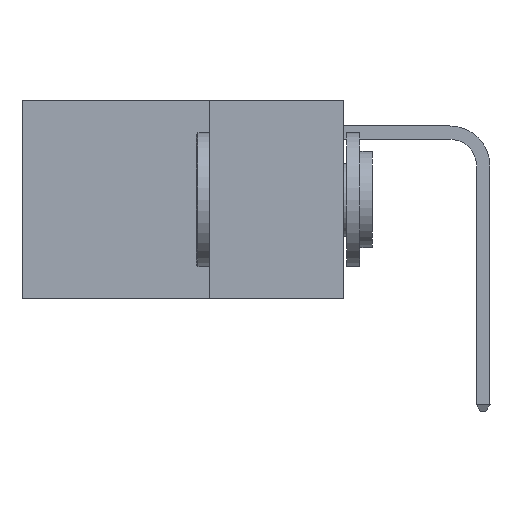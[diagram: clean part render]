
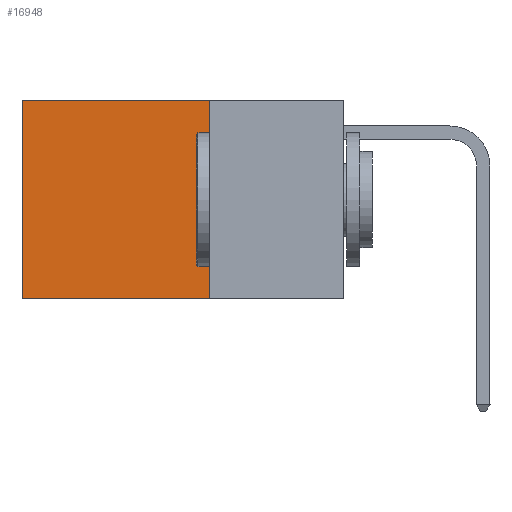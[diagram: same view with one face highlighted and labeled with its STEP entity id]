
A CAD part, left-side view. The second image highlights one B-rep face of the part: STEP entity #16948.
In plain terms, the highlighted planar face has unit normal (-1, 0, 0).
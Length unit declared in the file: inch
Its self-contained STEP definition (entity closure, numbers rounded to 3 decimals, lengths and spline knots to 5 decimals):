
#897 = EDGE_CURVE ( 'NONE', #18017, #7083, #15441, .T. ) ;
#962 = DIRECTION ( 'NONE',  ( 0., 0., -1. ) ) ;
#1536 = CARTESIAN_POINT ( 'NONE',  ( 0.2625, 0.25, -0.37 ) ) ;
#1868 = FACE_OUTER_BOUND ( 'NONE', #3925, .T. ) ;
#2265 = ORIENTED_EDGE ( 'NONE', *, *, #897, .F. ) ;
#2746 = DIRECTION ( 'NONE',  ( 0., 1., 0. ) ) ;
#3925 = EDGE_LOOP ( 'NONE', ( #17781, #7814, #2265, #12439 ) ) ;
#4164 = VERTEX_POINT ( 'NONE', #8130 ) ;
#4309 = VECTOR ( 'NONE', #13850, 39.37008 ) ;
#4644 = EDGE_CURVE ( 'NONE', #7083, #7301, #19339, .T. ) ;
#4795 = AXIS2_PLACEMENT_3D ( 'NONE', #13183, #19347, #19648 ) ;
#5491 = CARTESIAN_POINT ( 'NONE',  ( 0.2625, 0.25, 0. ) ) ;
#6534 = PLANE ( 'NONE',  #4795 ) ;
#7083 = VERTEX_POINT ( 'NONE', #1536 ) ;
#7301 = VERTEX_POINT ( 'NONE', #18677 ) ;
#7314 = CARTESIAN_POINT ( 'NONE',  ( 0.2625, 0.25, 0. ) ) ;
#7814 = ORIENTED_EDGE ( 'NONE', *, *, #4644, .F. ) ;
#7901 = CARTESIAN_POINT ( 'NONE',  ( 0.2625, 0.25, -0.37 ) ) ;
#8130 = CARTESIAN_POINT ( 'NONE',  ( 0.2625, 0.6, 0. ) ) ;
#9306 = LINE ( 'NONE', #17242, #10475 ) ;
#9488 = LINE ( 'NONE', #12964, #4309 ) ;
#9625 = EDGE_CURVE ( 'NONE', #4164, #7301, #9488, .T. ) ;
#10475 = VECTOR ( 'NONE', #2746, 39.37008 ) ;
#12439 = ORIENTED_EDGE ( 'NONE', *, *, #12889, .T. ) ;
#12889 = EDGE_CURVE ( 'NONE', #18017, #4164, #9306, .T. ) ;
#12964 = CARTESIAN_POINT ( 'NONE',  ( 0.2625, 0.6, 0. ) ) ;
#13183 = CARTESIAN_POINT ( 'NONE',  ( 0.2625, 0.25, 0. ) ) ;
#13433 = VECTOR ( 'NONE', #20813, 39.37008 ) ;
#13850 = DIRECTION ( 'NONE',  ( 0., 0., -1. ) ) ;
#14889 = VECTOR ( 'NONE', #962, 39.37008 ) ;
#15441 = LINE ( 'NONE', #7314, #14889 ) ;
#16948 = ADVANCED_FACE ( 'NONE', ( #1868 ), #6534, .F. ) ;
#17242 = CARTESIAN_POINT ( 'NONE',  ( 0.2625, 0.25, 0. ) ) ;
#17781 = ORIENTED_EDGE ( 'NONE', *, *, #9625, .T. ) ;
#18017 = VERTEX_POINT ( 'NONE', #5491 ) ;
#18677 = CARTESIAN_POINT ( 'NONE',  ( 0.2625, 0.6, -0.37 ) ) ;
#19339 = LINE ( 'NONE', #7901, #13433 ) ;
#19347 = DIRECTION ( 'NONE',  ( 1., 0., 0. ) ) ;
#19648 = DIRECTION ( 'NONE',  ( 0., 0., -1. ) ) ;
#20813 = DIRECTION ( 'NONE',  ( 0., 1., 0. ) ) ;
